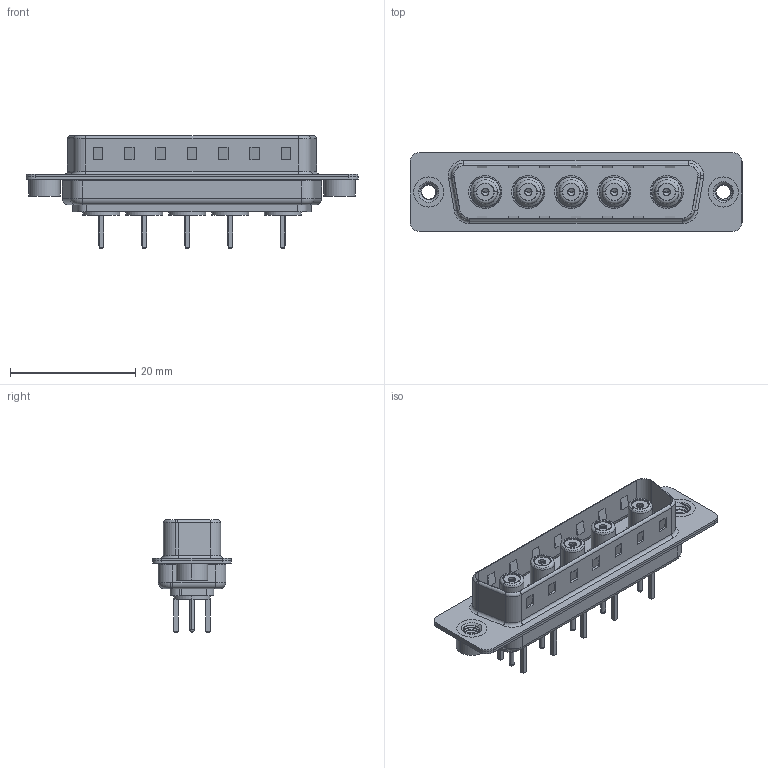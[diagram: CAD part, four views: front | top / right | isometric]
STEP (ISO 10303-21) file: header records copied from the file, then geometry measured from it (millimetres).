
FILE_DESCRIPTION (( 'STEP AP203' ), '1' );
FILE_NAME ('627-5W5-224-5TA.STEP', '2019-05-25T21:54:43', ( '' ), ( '' ), 'SwSTEP 2.0', 'SolidWorks 2016', '' );
FILE_SCHEMA (( 'CONFIG_CONTROL_DESIGN' ));
Length unit declared in the file: millimetre
Products named in the file (12): Co-Ax Jack Assy_S; Locking Collar; 627Combo Threaded Rivet_2; Socket_Str; 627Combo Housing_5W5; 627-5W5-224-5TA; 627Combo Shell Rear_25 Contacts; 627Combo Shell Front_25 Contacts; 627Combo Threaded Rivet_A; Co-Ax Jack_Straight PC Tail; Insulator Socket; Insulator Socket 2
Assembly tree (15 placements, depth 3):
  627-5W5-224-5TA
    627Combo Housing_5W5
    627Combo Shell Rear_25 Contacts
    627Combo Shell Front_25 Contacts
    627Combo Threaded Rivet_A
    Co-Ax Jack Assy_S  x5
      Co-Ax Jack_Straight PC Tail
      Insulator Socket
      Insulator Socket 2
      Locking Collar
      Socket_Str
    627Combo Threaded Rivet_2
Bounding box: 53 x 12.6 x 17.9 mm (x, y, z)
Volume: 2827.4 mm3; surface area: 8692.3 mm2
Topology: 30 solids, 30 shells, 930 faces, 2199 edges, 1380 vertices
Faces by surface type: plane 406, cylinder 373, torus 70, cone 55, bspline 16, sphere 10
Entity records: 19618 total; most frequent: CARTESIAN_POINT 5987, DIRECTION 2655, ORIENTED_EDGE 2490, EDGE_CURVE 1245, AXIS2_PLACEMENT_3D 984, VERTEX_POINT 788, LINE 687, VECTOR 687
